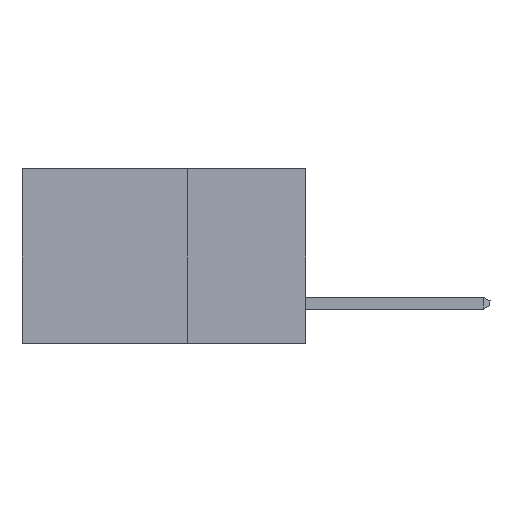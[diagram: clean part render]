
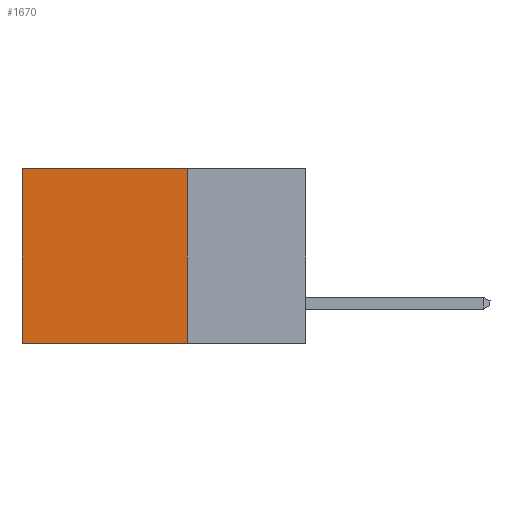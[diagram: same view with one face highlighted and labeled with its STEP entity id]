
A CAD part, left-side view. The second image highlights one B-rep face of the part: STEP entity #1670.
In plain terms, the highlighted planar face has unit normal (-1, 0, 0).
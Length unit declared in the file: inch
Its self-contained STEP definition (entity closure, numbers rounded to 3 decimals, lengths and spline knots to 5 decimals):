
#401 = VECTOR ( 'NONE', #4265, 39.37008 ) ;
#449 = CARTESIAN_POINT ( 'NONE',  ( 0.2615, 0.25, 0. ) ) ;
#820 = DIRECTION ( 'NONE',  ( 1., 0., 0. ) ) ;
#1107 = EDGE_CURVE ( 'NONE', #10943, #5704, #4166, .T. ) ;
#1666 = EDGE_CURVE ( 'NONE', #5704, #2021, #5309, .T. ) ;
#1670 = ADVANCED_FACE ( 'NONE', ( #1815 ), #11464, .F. ) ;
#1815 = FACE_OUTER_BOUND ( 'NONE', #10376, .T. ) ;
#1876 = CARTESIAN_POINT ( 'NONE',  ( 0.2615, 0.6, 0. ) ) ;
#2021 = VERTEX_POINT ( 'NONE', #6220 ) ;
#2241 = VECTOR ( 'NONE', #8529, 39.37008 ) ;
#3595 = CARTESIAN_POINT ( 'NONE',  ( 0.2615, 0.25, -0.37 ) ) ;
#3970 = VECTOR ( 'NONE', #10307, 39.37008 ) ;
#4008 = CARTESIAN_POINT ( 'NONE',  ( 0.2615, 0.25, 0. ) ) ;
#4166 = LINE ( 'NONE', #6889, #3970 ) ;
#4265 = DIRECTION ( 'NONE',  ( 0., 1., 0. ) ) ;
#4299 = LINE ( 'NONE', #11441, #4659 ) ;
#4325 = DIRECTION ( 'NONE',  ( 0., 0., -1. ) ) ;
#4407 = EDGE_CURVE ( 'NONE', #6853, #2021, #4299, .T. ) ;
#4422 = ORIENTED_EDGE ( 'NONE', *, *, #1107, .F. ) ;
#4642 = EDGE_CURVE ( 'NONE', #10943, #6853, #9234, .T. ) ;
#4659 = VECTOR ( 'NONE', #5984, 39.37008 ) ;
#4967 = ORIENTED_EDGE ( 'NONE', *, *, #4407, .T. ) ;
#5309 = LINE ( 'NONE', #8791, #401 ) ;
#5704 = VERTEX_POINT ( 'NONE', #3595 ) ;
#5971 = ORIENTED_EDGE ( 'NONE', *, *, #1666, .F. ) ;
#5984 = DIRECTION ( 'NONE',  ( 0., 0., -1. ) ) ;
#6063 = CARTESIAN_POINT ( 'NONE',  ( 0.2615, 0.25, -0.37 ) ) ;
#6220 = CARTESIAN_POINT ( 'NONE',  ( 0.2615, 0.6, -0.37 ) ) ;
#6853 = VERTEX_POINT ( 'NONE', #1876 ) ;
#6889 = CARTESIAN_POINT ( 'NONE',  ( 0.2615, 0.25, -0.37 ) ) ;
#7270 = AXIS2_PLACEMENT_3D ( 'NONE', #6063, #820, #4325 ) ;
#8043 = ORIENTED_EDGE ( 'NONE', *, *, #4642, .T. ) ;
#8529 = DIRECTION ( 'NONE',  ( 0., 1., 0. ) ) ;
#8791 = CARTESIAN_POINT ( 'NONE',  ( 0.2615, 0.25, -0.37 ) ) ;
#9234 = LINE ( 'NONE', #449, #2241 ) ;
#10307 = DIRECTION ( 'NONE',  ( 0., 0., -1. ) ) ;
#10376 = EDGE_LOOP ( 'NONE', ( #4967, #5971, #4422, #8043 ) ) ;
#10943 = VERTEX_POINT ( 'NONE', #4008 ) ;
#11441 = CARTESIAN_POINT ( 'NONE',  ( 0.2615, 0.6, -0.37 ) ) ;
#11464 = PLANE ( 'NONE',  #7270 ) ;
